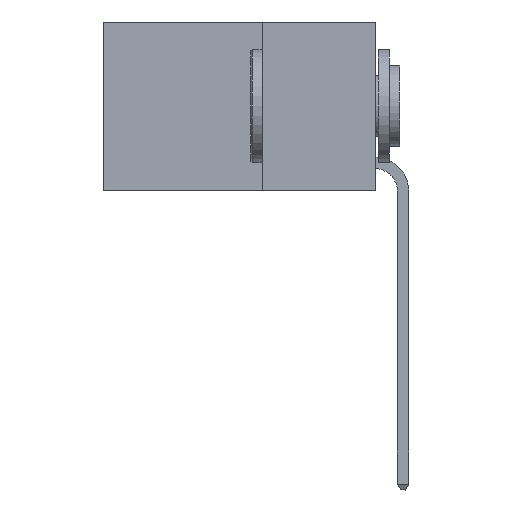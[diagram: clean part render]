
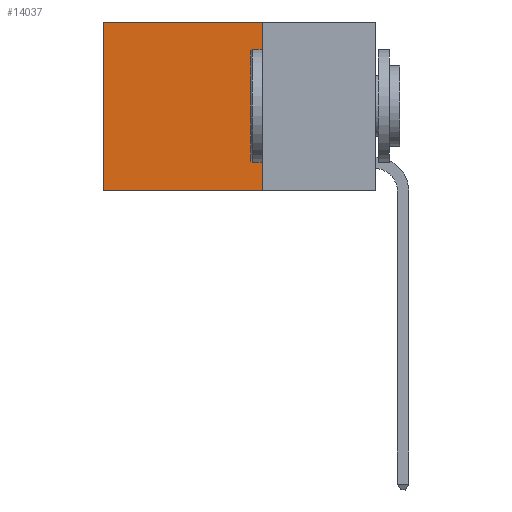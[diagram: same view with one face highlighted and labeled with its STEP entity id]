
A CAD part, left-side view. The second image highlights one B-rep face of the part: STEP entity #14037.
In plain terms, the highlighted planar face has unit normal (-1, 0, 0).
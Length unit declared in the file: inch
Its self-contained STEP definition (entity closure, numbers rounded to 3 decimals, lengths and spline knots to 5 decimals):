
#973 = EDGE_CURVE ( 'NONE', #19441, #10633, #1115, .T. ) ;
#1115 = LINE ( 'NONE', #18184, #5865 ) ;
#2404 = DIRECTION ( 'NONE',  ( 0., 1., 0. ) ) ;
#2944 = PLANE ( 'NONE',  #3731 ) ;
#3731 = AXIS2_PLACEMENT_3D ( 'NONE', #14783, #6984, #20783 ) ;
#4018 = ORIENTED_EDGE ( 'NONE', *, *, #973, .T. ) ;
#4078 = CARTESIAN_POINT ( 'NONE',  ( 0.2625, 0.6, 0. ) ) ;
#4474 = VECTOR ( 'NONE', #15900, 39.37008 ) ;
#4704 = ORIENTED_EDGE ( 'NONE', *, *, #23205, .F. ) ;
#5080 = EDGE_LOOP ( 'NONE', ( #23179, #4704, #9791, #4018 ) ) ;
#5263 = LINE ( 'NONE', #7883, #20426 ) ;
#5865 = VECTOR ( 'NONE', #2404, 39.37008 ) ;
#6676 = VECTOR ( 'NONE', #11209, 39.37008 ) ;
#6975 = CARTESIAN_POINT ( 'NONE',  ( 0.2625, 0.6, -0.37 ) ) ;
#6984 = DIRECTION ( 'NONE',  ( 1., 0., 0. ) ) ;
#7883 = CARTESIAN_POINT ( 'NONE',  ( 0.2625, 0.25, 0. ) ) ;
#9574 = CARTESIAN_POINT ( 'NONE',  ( 0.2625, 0.25, -0.37 ) ) ;
#9791 = ORIENTED_EDGE ( 'NONE', *, *, #14389, .F. ) ;
#10633 = VERTEX_POINT ( 'NONE', #24822 ) ;
#11209 = DIRECTION ( 'NONE',  ( 0., 1., 0. ) ) ;
#12697 = FACE_OUTER_BOUND ( 'NONE', #5080, .T. ) ;
#14037 = ADVANCED_FACE ( 'NONE', ( #12697 ), #2944, .F. ) ;
#14389 = EDGE_CURVE ( 'NONE', #19441, #16348, #5263, .T. ) ;
#14783 = CARTESIAN_POINT ( 'NONE',  ( 0.2625, 0.25, 0. ) ) ;
#15566 = LINE ( 'NONE', #4078, #4474 ) ;
#15900 = DIRECTION ( 'NONE',  ( 0., 0., -1. ) ) ;
#16348 = VERTEX_POINT ( 'NONE', #9574 ) ;
#16811 = LINE ( 'NONE', #23088, #6676 ) ;
#18184 = CARTESIAN_POINT ( 'NONE',  ( 0.2625, 0.25, 0. ) ) ;
#19441 = VERTEX_POINT ( 'NONE', #20257 ) ;
#20257 = CARTESIAN_POINT ( 'NONE',  ( 0.2625, 0.25, 0. ) ) ;
#20426 = VECTOR ( 'NONE', #23765, 39.37008 ) ;
#20783 = DIRECTION ( 'NONE',  ( 0., 0., -1. ) ) ;
#23088 = CARTESIAN_POINT ( 'NONE',  ( 0.2625, 0.25, -0.37 ) ) ;
#23179 = ORIENTED_EDGE ( 'NONE', *, *, #23501, .T. ) ;
#23205 = EDGE_CURVE ( 'NONE', #16348, #23810, #16811, .T. ) ;
#23501 = EDGE_CURVE ( 'NONE', #10633, #23810, #15566, .T. ) ;
#23765 = DIRECTION ( 'NONE',  ( 0., 0., -1. ) ) ;
#23810 = VERTEX_POINT ( 'NONE', #6975 ) ;
#24822 = CARTESIAN_POINT ( 'NONE',  ( 0.2625, 0.6, 0. ) ) ;
